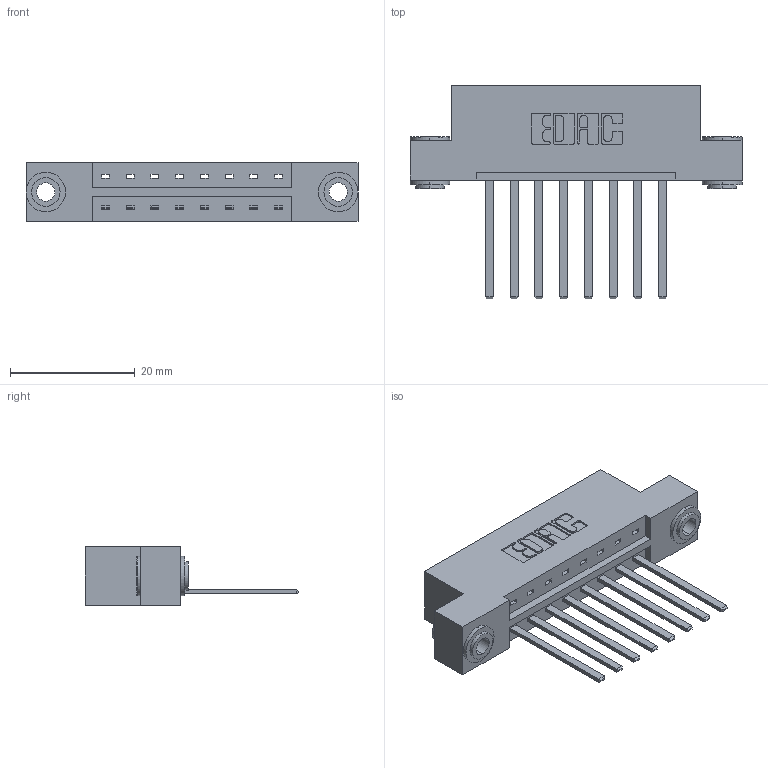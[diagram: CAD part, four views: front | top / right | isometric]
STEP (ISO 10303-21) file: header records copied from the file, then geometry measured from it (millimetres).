
FILE_DESCRIPTION (( 'STEP AP203' ), '1' );
FILE_NAME ('833-008-544-103.STEP', '2020-05-30T16:25:42', ( '' ), ( '' ), 'SwSTEP 2.0', 'SolidWorks 2020', '' );
FILE_SCHEMA (( 'CONFIG_CONTROL_DESIGN' ));
Length unit declared in the file: inch
Products named in the file (4): 833 Part_Flush - .156 Dia - TH; 345-250-002_345-250-002-102; 833-008-544-103; 345-292-001_345-293-144
Assembly tree (11 placements, depth 2):
  833-008-544-103
    833 Part_Flush - .156 Dia - TH
    345-292-001_345-293-144  x8
    345-250-002_345-250-002-102  x2
Bounding box: 53.24 x 34.3 x 9.4 mm (x, y, z)
Volume: 5176.9 mm3; surface area: 5907.6 mm2
Topology: 11 solids, 11 shells, 568 faces, 1651 edges, 1086 vertices
Faces by surface type: plane 384, cylinder 176, cone 8
Entity records: 9754 total; most frequent: CARTESIAN_POINT 1665, ORIENTED_EDGE 1602, DIRECTION 1503, EDGE_CURVE 801, VECTOR 653, LINE 653, VERTEX_POINT 530, AXIS2_PLACEMENT_3D 425
